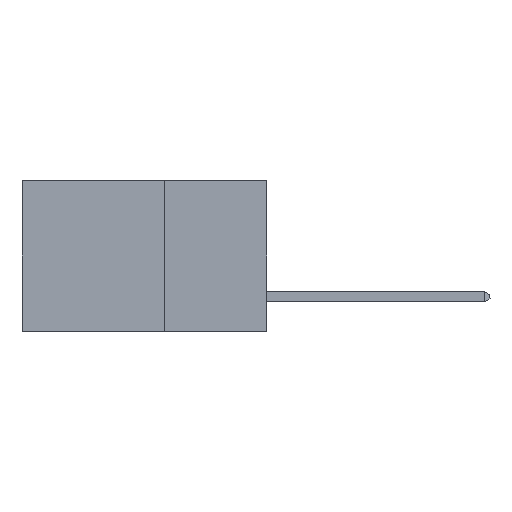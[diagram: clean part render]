
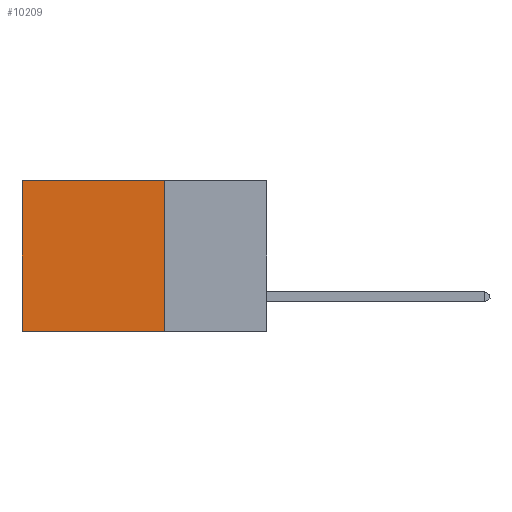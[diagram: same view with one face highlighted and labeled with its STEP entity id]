
A CAD part, left-side view. The second image highlights one B-rep face of the part: STEP entity #10209.
In plain terms, the highlighted planar face has unit normal (-1, 0, 0).
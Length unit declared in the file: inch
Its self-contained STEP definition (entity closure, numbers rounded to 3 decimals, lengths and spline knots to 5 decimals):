
#197 = LINE ( 'NONE', #13327, #2985 ) ;
#242 = DIRECTION ( 'NONE',  ( 0., 1., 0. ) ) ;
#2347 = PLANE ( 'NONE',  #4594 ) ;
#2763 = VERTEX_POINT ( 'NONE', #6618 ) ;
#2985 = VECTOR ( 'NONE', #4994, 39.37008 ) ;
#3385 = ORIENTED_EDGE ( 'NONE', *, *, #17951, .T. ) ;
#4594 = AXIS2_PLACEMENT_3D ( 'NONE', #5528, #12243, #15225 ) ;
#4727 = LINE ( 'NONE', #15566, #9721 ) ;
#4994 = DIRECTION ( 'NONE',  ( 0., 1., 0. ) ) ;
#5326 = LINE ( 'NONE', #16851, #9643 ) ;
#5528 = CARTESIAN_POINT ( 'NONE',  ( 0.2875, 0.25, 0. ) ) ;
#6052 = EDGE_CURVE ( 'NONE', #11915, #7899, #197, .T. ) ;
#6083 = ORIENTED_EDGE ( 'NONE', *, *, #16515, .T. ) ;
#6295 = EDGE_CURVE ( 'NONE', #16924, #11915, #4727, .T. ) ;
#6618 = CARTESIAN_POINT ( 'NONE',  ( 0.2875, 0.6, 0. ) ) ;
#7899 = VERTEX_POINT ( 'NONE', #17487 ) ;
#8732 = DIRECTION ( 'NONE',  ( 0., 0., -1. ) ) ;
#9643 = VECTOR ( 'NONE', #242, 39.37008 ) ;
#9721 = VECTOR ( 'NONE', #8732, 39.37008 ) ;
#9955 = CARTESIAN_POINT ( 'NONE',  ( 0.2875, 0.25, -0.37 ) ) ;
#10209 = ADVANCED_FACE ( 'NONE', ( #12573 ), #2347, .F. ) ;
#10473 = CARTESIAN_POINT ( 'NONE',  ( 0.2875, 0.25, 0. ) ) ;
#11103 = LINE ( 'NONE', #11461, #14654 ) ;
#11105 = ORIENTED_EDGE ( 'NONE', *, *, #6295, .F. ) ;
#11461 = CARTESIAN_POINT ( 'NONE',  ( 0.2875, 0.6, 0. ) ) ;
#11915 = VERTEX_POINT ( 'NONE', #9955 ) ;
#11924 = EDGE_LOOP ( 'NONE', ( #3385, #16349, #11105, #6083 ) ) ;
#12243 = DIRECTION ( 'NONE',  ( 1., 0., 0. ) ) ;
#12573 = FACE_OUTER_BOUND ( 'NONE', #11924, .T. ) ;
#13327 = CARTESIAN_POINT ( 'NONE',  ( 0.2875, 0.25, -0.37 ) ) ;
#14654 = VECTOR ( 'NONE', #16828, 39.37008 ) ;
#15225 = DIRECTION ( 'NONE',  ( 0., 0., -1. ) ) ;
#15566 = CARTESIAN_POINT ( 'NONE',  ( 0.2875, 0.25, 0. ) ) ;
#16349 = ORIENTED_EDGE ( 'NONE', *, *, #6052, .F. ) ;
#16515 = EDGE_CURVE ( 'NONE', #16924, #2763, #5326, .T. ) ;
#16828 = DIRECTION ( 'NONE',  ( 0., 0., -1. ) ) ;
#16851 = CARTESIAN_POINT ( 'NONE',  ( 0.2875, 0.25, 0. ) ) ;
#16924 = VERTEX_POINT ( 'NONE', #10473 ) ;
#17487 = CARTESIAN_POINT ( 'NONE',  ( 0.2875, 0.6, -0.37 ) ) ;
#17951 = EDGE_CURVE ( 'NONE', #2763, #7899, #11103, .T. ) ;
